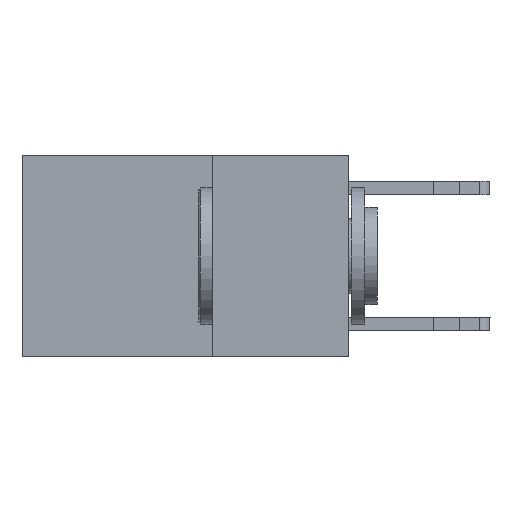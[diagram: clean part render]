
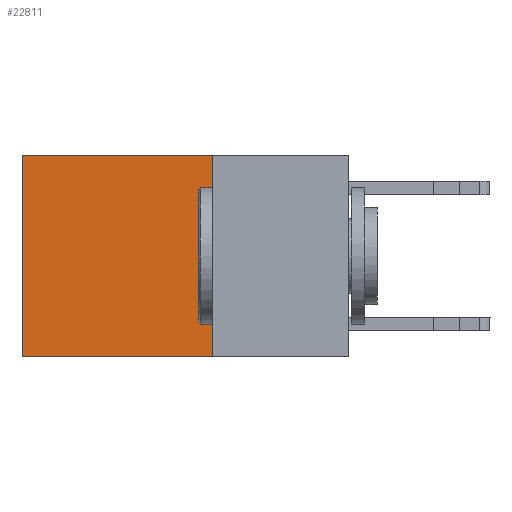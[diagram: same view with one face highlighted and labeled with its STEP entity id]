
A CAD part, left-side view. The second image highlights one B-rep face of the part: STEP entity #22811.
In plain terms, the highlighted planar face has unit normal (-1, 0, 0).
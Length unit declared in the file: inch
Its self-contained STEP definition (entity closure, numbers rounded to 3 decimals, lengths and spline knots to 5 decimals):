
#61 = ORIENTED_EDGE ( 'NONE', *, *, #12642, .F. ) ;
#286 = VECTOR ( 'NONE', #3489, 39.37008 ) ;
#458 = LINE ( 'NONE', #3029, #16633 ) ;
#950 = DIRECTION ( 'NONE',  ( 0., 0., -1. ) ) ;
#994 = AXIS2_PLACEMENT_3D ( 'NONE', #16366, #5762, #12538 ) ;
#1425 = EDGE_CURVE ( 'NONE', #7063, #6383, #3921, .T. ) ;
#1811 = FACE_OUTER_BOUND ( 'NONE', #21439, .T. ) ;
#3029 = CARTESIAN_POINT ( 'NONE',  ( 0.2625, 0.25, -0.37 ) ) ;
#3306 = CARTESIAN_POINT ( 'NONE',  ( 0.2625, 0.25, -0.37 ) ) ;
#3489 = DIRECTION ( 'NONE',  ( 0., 0., -1. ) ) ;
#3723 = PLANE ( 'NONE',  #994 ) ;
#3921 = LINE ( 'NONE', #12200, #18547 ) ;
#5762 = DIRECTION ( 'NONE',  ( 1., 0., 0. ) ) ;
#6383 = VERTEX_POINT ( 'NONE', #3306 ) ;
#7063 = VERTEX_POINT ( 'NONE', #13144 ) ;
#7109 = DIRECTION ( 'NONE',  ( 0., 1., 0. ) ) ;
#7298 = EDGE_CURVE ( 'NONE', #12278, #26794, #22122, .T. ) ;
#7914 = LINE ( 'NONE', #16593, #9706 ) ;
#9706 = VECTOR ( 'NONE', #14423, 39.37008 ) ;
#10214 = ORIENTED_EDGE ( 'NONE', *, *, #1425, .F. ) ;
#12200 = CARTESIAN_POINT ( 'NONE',  ( 0.2625, 0.25, 0. ) ) ;
#12278 = VERTEX_POINT ( 'NONE', #24154 ) ;
#12538 = DIRECTION ( 'NONE',  ( 0., 0., -1. ) ) ;
#12642 = EDGE_CURVE ( 'NONE', #6383, #26794, #458, .T. ) ;
#13144 = CARTESIAN_POINT ( 'NONE',  ( 0.2625, 0.25, 0. ) ) ;
#13170 = ORIENTED_EDGE ( 'NONE', *, *, #7298, .T. ) ;
#14358 = CARTESIAN_POINT ( 'NONE',  ( 0.2625, 0.6, 0. ) ) ;
#14423 = DIRECTION ( 'NONE',  ( 0., 1., 0. ) ) ;
#16366 = CARTESIAN_POINT ( 'NONE',  ( 0.2625, 0.25, 0. ) ) ;
#16593 = CARTESIAN_POINT ( 'NONE',  ( 0.2625, 0.25, 0. ) ) ;
#16633 = VECTOR ( 'NONE', #7109, 39.37008 ) ;
#17642 = ORIENTED_EDGE ( 'NONE', *, *, #23218, .T. ) ;
#18547 = VECTOR ( 'NONE', #950, 39.37008 ) ;
#19671 = CARTESIAN_POINT ( 'NONE',  ( 0.2625, 0.6, -0.37 ) ) ;
#21439 = EDGE_LOOP ( 'NONE', ( #13170, #61, #10214, #17642 ) ) ;
#22122 = LINE ( 'NONE', #14358, #286 ) ;
#22811 = ADVANCED_FACE ( 'NONE', ( #1811 ), #3723, .F. ) ;
#23218 = EDGE_CURVE ( 'NONE', #7063, #12278, #7914, .T. ) ;
#24154 = CARTESIAN_POINT ( 'NONE',  ( 0.2625, 0.6, 0. ) ) ;
#26794 = VERTEX_POINT ( 'NONE', #19671 ) ;
